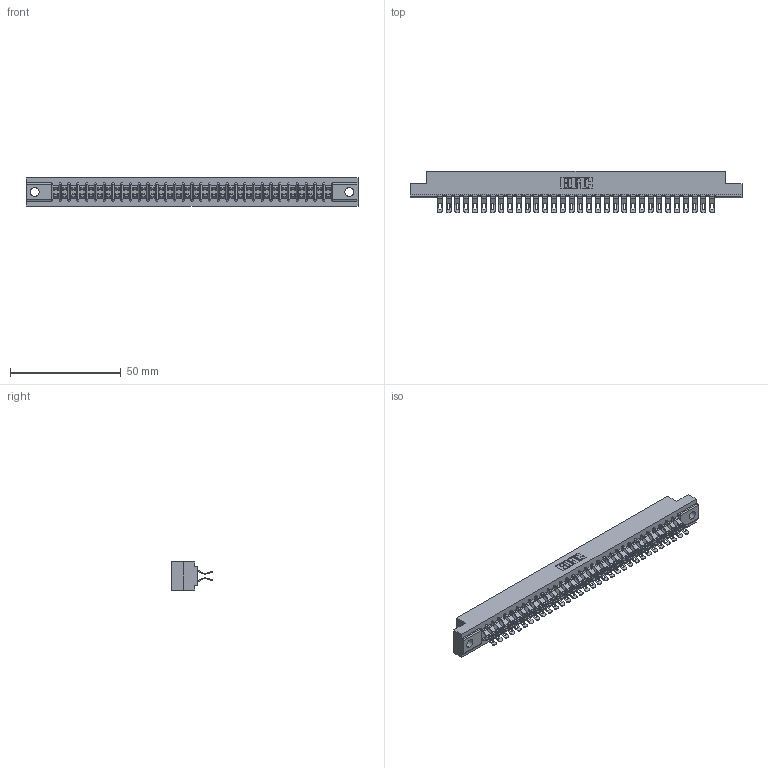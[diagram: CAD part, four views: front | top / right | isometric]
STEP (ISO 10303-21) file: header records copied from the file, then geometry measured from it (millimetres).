
FILE_DESCRIPTION (( 'STEP AP203' ), '1' );
FILE_NAME ('307-064-555-204.STEP', '2019-09-06T16:56:13', ( '' ), ( '' ), 'SwSTEP 2.0', 'SolidWorks 2016', '' );
FILE_SCHEMA (( 'CONFIG_CONTROL_DESIGN' ));
Length unit declared in the file: inch
Products named in the file (3): 307 Part_.156 Dia Mounting Holes; 307-064-555-204; 307-290-001_555
Assembly tree (65 placements, depth 2):
  307-064-555-204
    307 Part_.156 Dia Mounting Holes
    307-290-001_555  x64
Bounding box: 149.81 x 18.75 x 12.7 mm (x, y, z)
Volume: 15944.3 mm3; surface area: 20198.7 mm2
Topology: 65 solids, 65 shells, 4069 faces, 11943 edges, 7786 vertices
Faces by surface type: plane 2260, cylinder 1743, sphere 66
Entity records: 30645 total; most frequent: CARTESIAN_POINT 5026, ORIENTED_EDGE 4980, DIRECTION 4926, EDGE_CURVE 2490, LINE 1902, VECTOR 1902, VERTEX_POINT 1612, AXIS2_PLACEMENT_3D 1512
